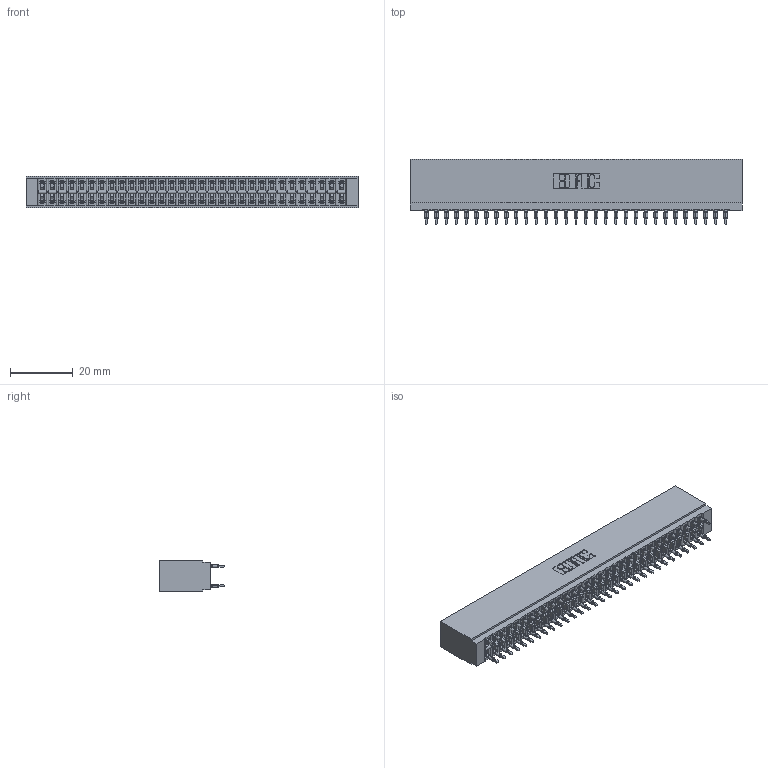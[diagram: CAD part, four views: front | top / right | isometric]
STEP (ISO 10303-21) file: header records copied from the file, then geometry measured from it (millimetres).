
FILE_DESCRIPTION (( 'STEP AP203' ), '1' );
FILE_NAME ('746-062-560-201.STEP', '2026-03-04T13:39:03', ( '' ), ( '' ), 'SwSTEP 2.0', 'SolidWorks 2023', '' );
FILE_SCHEMA (( 'CONFIG_CONTROL_DESIGN' ));
Length unit declared in the file: millimetre
Products named in the file (3): 746 Part_.515 Slot Depth - 01; 746-062-560-201; 746-292-001_560
Assembly tree (63 placements, depth 2):
  746-062-560-201
    746 Part_.515 Slot Depth - 01
    746-292-001_560  x62
Bounding box: 105.66 x 20.82 x 9.91 mm (x, y, z)
Volume: 11611.6 mm3; surface area: 19435.8 mm2
Topology: 63 solids, 63 shells, 5956 faces, 16569 edges, 10622 vertices
Faces by surface type: plane 2969, cylinder 1375, bspline 1240, torus 372
Entity records: 49578 total; most frequent: CARTESIAN_POINT 9949, ORIENTED_EDGE 8494, DIRECTION 7117, EDGE_CURVE 4247, LINE 3745, VECTOR 3745, VERTEX_POINT 2814, AXIS2_PLACEMENT_3D 1686
